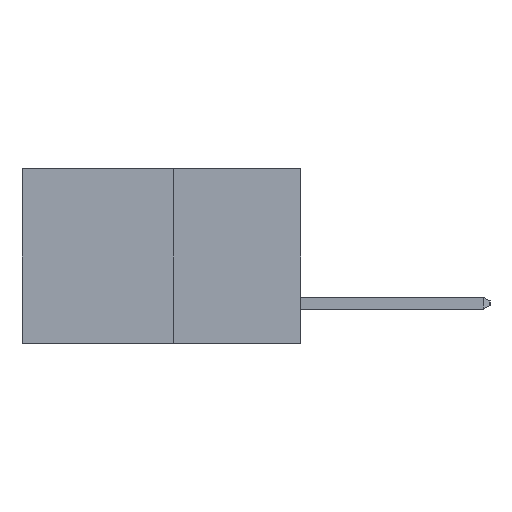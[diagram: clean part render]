
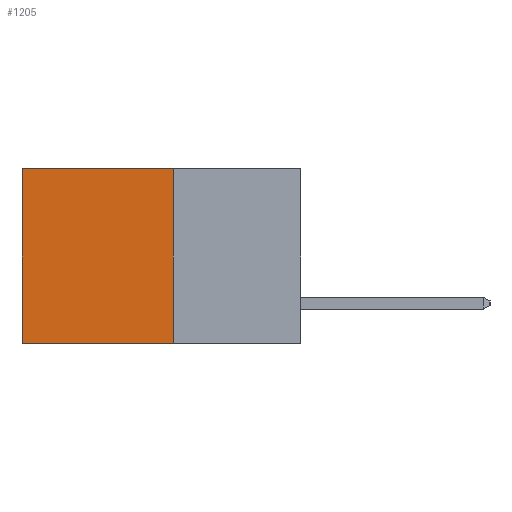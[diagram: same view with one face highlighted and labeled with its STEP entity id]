
A CAD part, left-side view. The second image highlights one B-rep face of the part: STEP entity #1205.
In plain terms, the highlighted planar face has unit normal (-1, 0, 0).
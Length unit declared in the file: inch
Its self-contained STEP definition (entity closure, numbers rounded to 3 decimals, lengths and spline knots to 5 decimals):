
#699 = ORIENTED_EDGE ( 'NONE', *, *, #12415, .T. ) ;
#1133 = CARTESIAN_POINT ( 'NONE',  ( 0.277, 0.27, -0.37 ) ) ;
#1205 = ADVANCED_FACE ( 'NONE', ( #10884 ), #10128, .F. ) ;
#1359 = DIRECTION ( 'NONE',  ( 1., 0., 0. ) ) ;
#1920 = LINE ( 'NONE', #8018, #18790 ) ;
#3128 = DIRECTION ( 'NONE',  ( 0., 0., -1. ) ) ;
#3513 = VERTEX_POINT ( 'NONE', #5586 ) ;
#3567 = CARTESIAN_POINT ( 'NONE',  ( 0.277, 0.27, -0.37 ) ) ;
#3905 = ORIENTED_EDGE ( 'NONE', *, *, #16530, .F. ) ;
#5201 = EDGE_CURVE ( 'NONE', #16133, #3513, #21154, .T. ) ;
#5586 = CARTESIAN_POINT ( 'NONE',  ( 0.277, 0.59, 0. ) ) ;
#6063 = DIRECTION ( 'NONE',  ( 0., 0., -1. ) ) ;
#6244 = ORIENTED_EDGE ( 'NONE', *, *, #5201, .T. ) ;
#6435 = CARTESIAN_POINT ( 'NONE',  ( 0.277, 0.59, -0.37 ) ) ;
#6469 = DIRECTION ( 'NONE',  ( 0., 1., 0. ) ) ;
#7518 = AXIS2_PLACEMENT_3D ( 'NONE', #1133, #1359, #6063 ) ;
#7908 = EDGE_LOOP ( 'NONE', ( #699, #3905, #17526, #6244 ) ) ;
#8018 = CARTESIAN_POINT ( 'NONE',  ( 0.277, 0.59, -0.37 ) ) ;
#8833 = LINE ( 'NONE', #8860, #13135 ) ;
#8860 = CARTESIAN_POINT ( 'NONE',  ( 0.277, 0.27, -0.37 ) ) ;
#10128 = PLANE ( 'NONE',  #7518 ) ;
#10495 = VERTEX_POINT ( 'NONE', #6435 ) ;
#10671 = VERTEX_POINT ( 'NONE', #3567 ) ;
#10739 = LINE ( 'NONE', #17099, #18900 ) ;
#10884 = FACE_OUTER_BOUND ( 'NONE', #7908, .T. ) ;
#11075 = CARTESIAN_POINT ( 'NONE',  ( 0.277, 0.27, 0. ) ) ;
#12415 = EDGE_CURVE ( 'NONE', #3513, #10495, #1920, .T. ) ;
#13135 = VECTOR ( 'NONE', #18648, 39.37008 ) ;
#13445 = EDGE_CURVE ( 'NONE', #16133, #10671, #10739, .T. ) ;
#16133 = VERTEX_POINT ( 'NONE', #11075 ) ;
#16236 = CARTESIAN_POINT ( 'NONE',  ( 0.277, 0.27, 0. ) ) ;
#16530 = EDGE_CURVE ( 'NONE', #10671, #10495, #8833, .T. ) ;
#16830 = VECTOR ( 'NONE', #6469, 39.37008 ) ;
#17099 = CARTESIAN_POINT ( 'NONE',  ( 0.277, 0.27, -0.37 ) ) ;
#17526 = ORIENTED_EDGE ( 'NONE', *, *, #13445, .F. ) ;
#18648 = DIRECTION ( 'NONE',  ( 0., 1., 0. ) ) ;
#18748 = DIRECTION ( 'NONE',  ( 0., 0., -1. ) ) ;
#18790 = VECTOR ( 'NONE', #3128, 39.37008 ) ;
#18900 = VECTOR ( 'NONE', #18748, 39.37008 ) ;
#21154 = LINE ( 'NONE', #16236, #16830 ) ;
